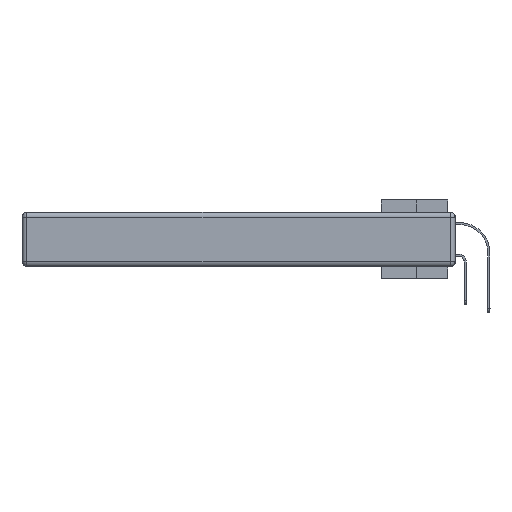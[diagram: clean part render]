
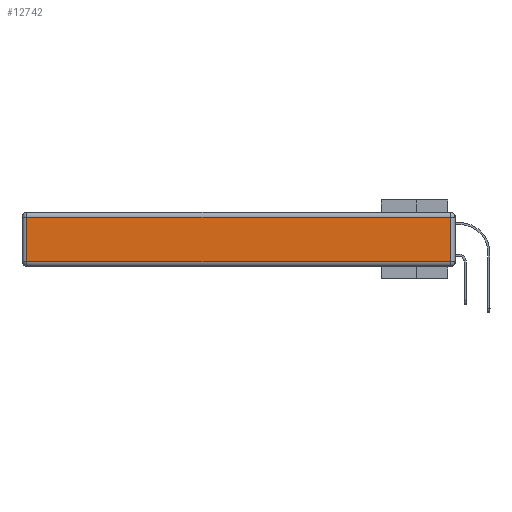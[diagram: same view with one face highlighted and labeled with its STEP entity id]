
A CAD part, left-side view. The second image highlights one B-rep face of the part: STEP entity #12742.
In plain terms, the highlighted planar face has unit normal (-1, 0, 0).
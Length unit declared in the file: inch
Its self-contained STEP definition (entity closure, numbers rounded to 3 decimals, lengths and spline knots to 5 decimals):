
#517 = LINE ( 'NONE', #12418, #21709 ) ;
#1071 = CARTESIAN_POINT ( 'NONE',  ( 0., 0.03, -0.03 ) ) ;
#2892 = DIRECTION ( 'NONE',  ( 0., 1., 0. ) ) ;
#3891 = DIRECTION ( 'NONE',  ( 0., 0., 1. ) ) ;
#5137 = ORIENTED_EDGE ( 'NONE', *, *, #25797, .T. ) ;
#5185 = ORIENTED_EDGE ( 'NONE', *, *, #6339, .T. ) ;
#5295 = AXIS2_PLACEMENT_3D ( 'NONE', #8281, #20410, #14611 ) ;
#5470 = LINE ( 'NONE', #33306, #35902 ) ;
#6086 = ORIENTED_EDGE ( 'NONE', *, *, #15110, .T. ) ;
#6339 = EDGE_CURVE ( 'NONE', #18361, #17162, #517, .T. ) ;
#6833 = DIRECTION ( 'NONE',  ( 0., -1., 0. ) ) ;
#8281 = CARTESIAN_POINT ( 'NONE',  ( 0., 0., -0.343 ) ) ;
#11045 = CARTESIAN_POINT ( 'NONE',  ( 0., 0.03, -0.313 ) ) ;
#11268 = VECTOR ( 'NONE', #2892, 39.37008 ) ;
#12193 = CARTESIAN_POINT ( 'NONE',  ( 0., 2.75, -0.03 ) ) ;
#12418 = CARTESIAN_POINT ( 'NONE',  ( 0., 0.03, -0.343 ) ) ;
#12742 = ADVANCED_FACE ( 'NONE', ( #30148 ), #32923, .T. ) ;
#12991 = LINE ( 'NONE', #30898, #13316 ) ;
#13316 = VECTOR ( 'NONE', #6833, 39.37008 ) ;
#13618 = VERTEX_POINT ( 'NONE', #17514 ) ;
#14611 = DIRECTION ( 'NONE',  ( 0., 0., 1. ) ) ;
#15069 = CARTESIAN_POINT ( 'NONE',  ( 0., 2.72, -0.03 ) ) ;
#15110 = EDGE_CURVE ( 'NONE', #17162, #35904, #27736, .T. ) ;
#17162 = VERTEX_POINT ( 'NONE', #1071 ) ;
#17514 = CARTESIAN_POINT ( 'NONE',  ( 0., 2.72, -0.313 ) ) ;
#17586 = DIRECTION ( 'NONE',  ( 0., 0., -1. ) ) ;
#18361 = VERTEX_POINT ( 'NONE', #11045 ) ;
#20410 = DIRECTION ( 'NONE',  ( -1., 0., 0. ) ) ;
#21027 = ORIENTED_EDGE ( 'NONE', *, *, #33723, .T. ) ;
#21709 = VECTOR ( 'NONE', #3891, 39.37008 ) ;
#22231 = EDGE_LOOP ( 'NONE', ( #21027, #5185, #6086, #5137 ) ) ;
#25797 = EDGE_CURVE ( 'NONE', #35904, #13618, #5470, .T. ) ;
#27736 = LINE ( 'NONE', #12193, #11268 ) ;
#30148 = FACE_OUTER_BOUND ( 'NONE', #22231, .T. ) ;
#30898 = CARTESIAN_POINT ( 'NONE',  ( 0., 0., -0.313 ) ) ;
#32923 = PLANE ( 'NONE',  #5295 ) ;
#33306 = CARTESIAN_POINT ( 'NONE',  ( 0., 2.72, -0.343 ) ) ;
#33723 = EDGE_CURVE ( 'NONE', #13618, #18361, #12991, .T. ) ;
#35902 = VECTOR ( 'NONE', #17586, 39.37008 ) ;
#35904 = VERTEX_POINT ( 'NONE', #15069 ) ;
